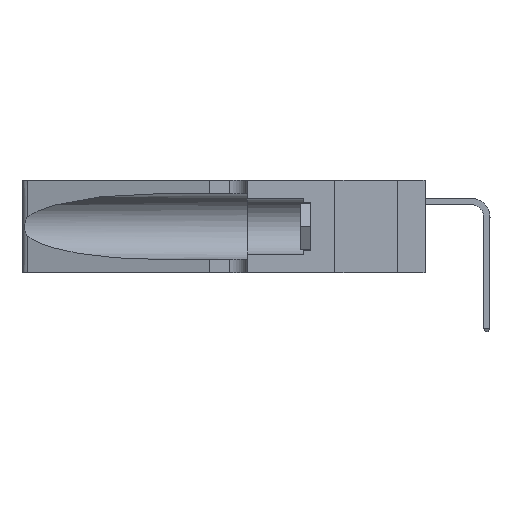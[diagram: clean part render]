
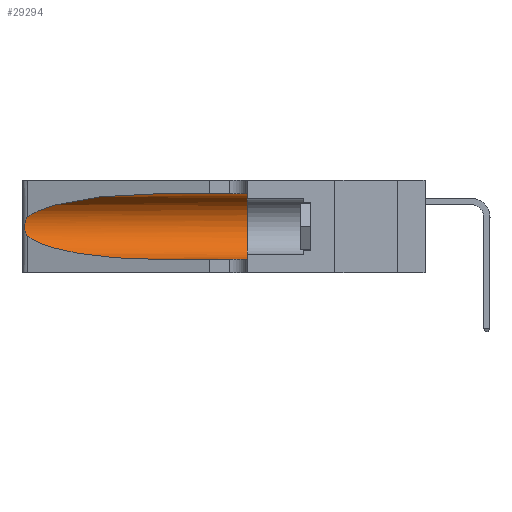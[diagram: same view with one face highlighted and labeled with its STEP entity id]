
A CAD part, left-side view. The second image highlights one B-rep face of the part: STEP entity #29294.
In plain terms, the highlighted cylindrical face has radius 3.308 mm (diameter 6.617 mm), a partial arc.
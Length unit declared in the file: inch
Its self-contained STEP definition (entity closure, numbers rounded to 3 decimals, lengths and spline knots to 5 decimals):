
#995 = CARTESIAN_POINT ( 'NONE',  ( 0.2373, 1.15595, 0.08982 ) ) ;
#1424 = CARTESIAN_POINT ( 'NONE',  ( 0.25787, 1.23484, 0.2124 ) ) ;
#2455 = CARTESIAN_POINT ( 'NONE',  ( 0.2373, 1.15595, 0.28018 ) ) ;
#3405 = CYLINDRICAL_SURFACE ( 'NONE', #16232, 0.13025 ) ;
#3406 = ORIENTED_EDGE ( 'NONE', *, *, #10500, .F. ) ;
#3915 = LINE ( 'NONE', #27961, #29153 ) ;
#4165 = B_SPLINE_CURVE_WITH_KNOTS ( 'NONE', 3,
 ( #11225, #30929, #21223, #1424, #24533, #4761, #27828, #8058, #31064, #11374, #34395, #14716, #37698, #18036 ),
 .UNSPECIFIED., .F., .F.,
 ( 4, 2, 2, 2, 2, 2, 4 ),
 ( 0., 0.00027, 0.00053, 0.00107, 0.0016, 0.00187, 0.00214 ),
 .UNSPECIFIED. ) ;
#4543 =( BOUNDED_CURVE ( )  B_SPLINE_CURVE ( 3, ( #20926, #995, #7771, #30787 ),
 .UNSPECIFIED., .F., .F. ) 
 B_SPLINE_CURVE_WITH_KNOTS ( ( 4, 4 ),
 ( 3.44316, 4.71239 ),
 .UNSPECIFIED. ) 
 CURVE ( )  GEOMETRIC_REPRESENTATION_ITEM ( )  RATIONAL_B_SPLINE_CURVE ( ( 1., 0.87, 0.87, 1. ) ) 
 REPRESENTATION_ITEM ( '' )  );
#4684 = DIRECTION ( 'NONE',  ( 0., 1., 0. ) ) ;
#4761 = CARTESIAN_POINT ( 'NONE',  ( 0.26018, 1.23835, 0.19895 ) ) ;
#5168 = CARTESIAN_POINT ( 'NONE',  ( 0.25487, 1.22718, 0.22369 ) ) ;
#5548 = LINE ( 'NONE', #19310, #30766 ) ;
#6319 = EDGE_CURVE ( 'NONE', #34419, #33219, #3915, .T. ) ;
#6369 = VERTEX_POINT ( 'NONE', #5168 ) ;
#7181 = VERTEX_POINT ( 'NONE', #15951 ) ;
#7715 = ORIENTED_EDGE ( 'NONE', *, *, #16471, .T. ) ;
#7771 = CARTESIAN_POINT ( 'NONE',  ( 0.18966, 0.96281, 0.05475 ) ) ;
#8058 = CARTESIAN_POINT ( 'NONE',  ( 0.26075, 1.23896, 0.178 ) ) ;
#8652 = VERTEX_POINT ( 'NONE', #36790 ) ;
#10478 =( BOUNDED_CURVE ( )  B_SPLINE_CURVE ( 3, ( #18935, #41910, #2455, #25549 ),
 .UNSPECIFIED., .F., .T. ) 
 B_SPLINE_CURVE_WITH_KNOTS ( ( 4, 4 ),
 ( 1.5708, 2.84003 ),
 .UNSPECIFIED. ) 
 CURVE ( )  GEOMETRIC_REPRESENTATION_ITEM ( )  RATIONAL_B_SPLINE_CURVE ( ( 1., 0.87, 0.87, 1. ) ) 
 REPRESENTATION_ITEM ( '' )  );
#10500 = EDGE_CURVE ( 'NONE', #33219, #22252, #14055, .T. ) ;
#11225 = CARTESIAN_POINT ( 'NONE',  ( 0.25487, 1.22718, 0.22369 ) ) ;
#11374 = CARTESIAN_POINT ( 'NONE',  ( 0.25856, 1.23593, 0.16098 ) ) ;
#13222 = FACE_OUTER_BOUND ( 'NONE', #21723, .T. ) ;
#14055 = CIRCLE ( 'NONE', #14609, 0.13025 ) ;
#14609 = AXIS2_PLACEMENT_3D ( 'NONE', #24456, #4684, #27749 ) ;
#14716 = CARTESIAN_POINT ( 'NONE',  ( 0.25639, 1.23186, 0.15144 ) ) ;
#15951 = CARTESIAN_POINT ( 'NONE',  ( 0.25487, 1.22718, 0.14631 ) ) ;
#16232 = AXIS2_PLACEMENT_3D ( 'NONE', #29467, #37395, #23065 ) ;
#16471 = EDGE_CURVE ( 'NONE', #7181, #8652, #4543, .T. ) ;
#16770 = EDGE_CURVE ( 'NONE', #8652, #22252, #5548, .T. ) ;
#18036 = CARTESIAN_POINT ( 'NONE',  ( 0.25487, 1.22718, 0.14631 ) ) ;
#18935 = CARTESIAN_POINT ( 'NONE',  ( 0.1305, 0.72297, 0.31525 ) ) ;
#19310 = CARTESIAN_POINT ( 'NONE',  ( 0.1305, 1.61858, 0.05475 ) ) ;
#20926 = CARTESIAN_POINT ( 'NONE',  ( 0.25487, 1.22718, 0.14631 ) ) ;
#21007 = ORIENTED_EDGE ( 'NONE', *, *, #6319, .F. ) ;
#21223 = CARTESIAN_POINT ( 'NONE',  ( 0.25639, 1.23184, 0.21858 ) ) ;
#21723 = EDGE_LOOP ( 'NONE', ( #33224, #34435, #7715, #34630, #3406, #21007 ) ) ;
#22252 = VERTEX_POINT ( 'NONE', #36184 ) ;
#23065 = DIRECTION ( 'NONE',  ( 0., 0., -1. ) ) ;
#24456 = CARTESIAN_POINT ( 'NONE',  ( 0.1305, 0.35, 0.185 ) ) ;
#24533 = CARTESIAN_POINT ( 'NONE',  ( 0.25854, 1.2359, 0.20912 ) ) ;
#25007 = EDGE_CURVE ( 'NONE', #6369, #7181, #4165, .T. ) ;
#25549 = CARTESIAN_POINT ( 'NONE',  ( 0.25487, 1.22718, 0.22369 ) ) ;
#27749 = DIRECTION ( 'NONE',  ( 0., 0., 1. ) ) ;
#27828 = CARTESIAN_POINT ( 'NONE',  ( 0.26075, 1.23896, 0.19203 ) ) ;
#27961 = CARTESIAN_POINT ( 'NONE',  ( 0.1305, 1.61858, 0.31525 ) ) ;
#28447 = EDGE_CURVE ( 'NONE', #34419, #6369, #10478, .T. ) ;
#29153 = VECTOR ( 'NONE', #34534, 39.37008 ) ;
#29294 = ADVANCED_FACE ( 'NONE', ( #13222 ), #3405, .F. ) ;
#29467 = CARTESIAN_POINT ( 'NONE',  ( 0.1305, 1.61858, 0.185 ) ) ;
#30713 = CARTESIAN_POINT ( 'NONE',  ( 0.1305, 0.72297, 0.31525 ) ) ;
#30766 = VECTOR ( 'NONE', #38982, 39.37008 ) ;
#30787 = CARTESIAN_POINT ( 'NONE',  ( 0.1305, 0.72297, 0.05475 ) ) ;
#30929 = CARTESIAN_POINT ( 'NONE',  ( 0.25555, 1.22994, 0.2215 ) ) ;
#31064 = CARTESIAN_POINT ( 'NONE',  ( 0.26017, 1.23833, 0.17102 ) ) ;
#31380 = CARTESIAN_POINT ( 'NONE',  ( 0.1305, 0.35, 0.31525 ) ) ;
#33219 = VERTEX_POINT ( 'NONE', #31380 ) ;
#33224 = ORIENTED_EDGE ( 'NONE', *, *, #28447, .T. ) ;
#34395 = CARTESIAN_POINT ( 'NONE',  ( 0.25789, 1.23486, 0.15765 ) ) ;
#34419 = VERTEX_POINT ( 'NONE', #30713 ) ;
#34435 = ORIENTED_EDGE ( 'NONE', *, *, #25007, .T. ) ;
#34534 = DIRECTION ( 'NONE',  ( 0., -1., 0. ) ) ;
#34630 = ORIENTED_EDGE ( 'NONE', *, *, #16770, .T. ) ;
#36184 = CARTESIAN_POINT ( 'NONE',  ( 0.1305, 0.35, 0.05475 ) ) ;
#36790 = CARTESIAN_POINT ( 'NONE',  ( 0.1305, 0.72297, 0.05475 ) ) ;
#37395 = DIRECTION ( 'NONE',  ( 0., -1., 0. ) ) ;
#37698 = CARTESIAN_POINT ( 'NONE',  ( 0.25555, 1.22993, 0.14849 ) ) ;
#38982 = DIRECTION ( 'NONE',  ( 0., -1., 0. ) ) ;
#41910 = CARTESIAN_POINT ( 'NONE',  ( 0.18966, 0.96281, 0.31525 ) ) ;
